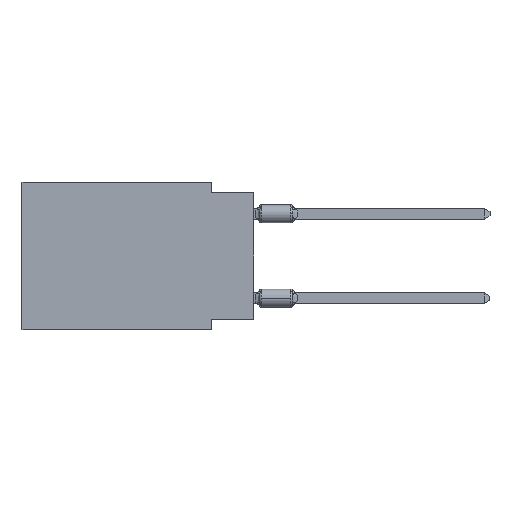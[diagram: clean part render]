
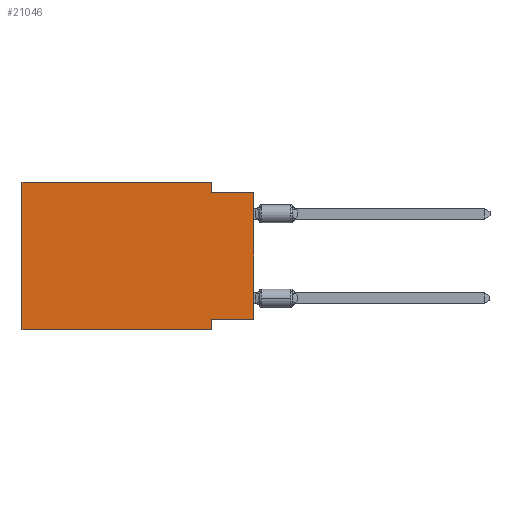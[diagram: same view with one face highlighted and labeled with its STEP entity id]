
A CAD part, left-side view. The second image highlights one B-rep face of the part: STEP entity #21046.
In plain terms, the highlighted planar face has unit normal (-1, 0, 0).
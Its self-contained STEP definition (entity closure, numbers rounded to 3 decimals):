
#267 = DIRECTION ( 'NONE',  ( 0., 1., 0. ) ) ;
#552 = EDGE_CURVE ( 'NONE', #5822, #3791, #19128, .T. ) ;
#1053 = LINE ( 'NONE', #17339, #16073 ) ;
#1590 = LINE ( 'NONE', #17991, #16207 ) ;
#1640 = VERTEX_POINT ( 'NONE', #14277 ) ;
#1796 = EDGE_CURVE ( 'NONE', #1640, #10874, #2358, .T. ) ;
#1816 = EDGE_CURVE ( 'NONE', #7917, #1640, #7277, .T. ) ;
#1916 = ORIENTED_EDGE ( 'NONE', *, *, #3583, .F. ) ;
#2358 = LINE ( 'NONE', #20168, #6768 ) ;
#2678 = VECTOR ( 'NONE', #6138, 1000. ) ;
#3006 = ORIENTED_EDGE ( 'NONE', *, *, #10089, .F. ) ;
#3583 = EDGE_CURVE ( 'NONE', #10874, #5408, #1053, .T. ) ;
#3791 = VERTEX_POINT ( 'NONE', #18504 ) ;
#3959 = FACE_OUTER_BOUND ( 'NONE', #9034, .T. ) ;
#4939 = LINE ( 'NONE', #11391, #18967 ) ;
#5405 = VECTOR ( 'NONE', #8885, 1000. ) ;
#5408 = VERTEX_POINT ( 'NONE', #6044 ) ;
#5555 = CARTESIAN_POINT ( 'NONE',  ( 0., 13.97, 0. ) ) ;
#5822 = VERTEX_POINT ( 'NONE', #7434 ) ;
#5949 = VECTOR ( 'NONE', #267, 1000. ) ;
#6044 = CARTESIAN_POINT ( 'NONE',  ( 0., 2.54, -0.635 ) ) ;
#6049 = CARTESIAN_POINT ( 'NONE',  ( 0., 2.54, -8.255 ) ) ;
#6138 = DIRECTION ( 'NONE',  ( 0., 0., 1. ) ) ;
#6193 = DIRECTION ( 'NONE',  ( 1., 0., 0. ) ) ;
#6768 = VECTOR ( 'NONE', #18866, 1000. ) ;
#6989 = VERTEX_POINT ( 'NONE', #12054 ) ;
#7099 = ORIENTED_EDGE ( 'NONE', *, *, #16585, .T. ) ;
#7277 = LINE ( 'NONE', #5555, #5405 ) ;
#7434 = CARTESIAN_POINT ( 'NONE',  ( 0., 0., -8.255 ) ) ;
#7748 = CARTESIAN_POINT ( 'NONE',  ( 0., 0., 0. ) ) ;
#7917 = VERTEX_POINT ( 'NONE', #17046 ) ;
#8117 = DIRECTION ( 'NONE',  ( 0., 0., -1. ) ) ;
#8775 = CARTESIAN_POINT ( 'NONE',  ( 0., 2.54, 0. ) ) ;
#8819 = LINE ( 'NONE', #11829, #5949 ) ;
#8885 = DIRECTION ( 'NONE',  ( 0., 0., 1. ) ) ;
#9034 = EDGE_LOOP ( 'NONE', ( #11129, #19531, #1916, #21090, #13071, #7099, #3006, #9657 ) ) ;
#9657 = ORIENTED_EDGE ( 'NONE', *, *, #12760, .F. ) ;
#10089 = EDGE_CURVE ( 'NONE', #17240, #6989, #1590, .T. ) ;
#10495 = PLANE ( 'NONE',  #18399 ) ;
#10874 = VERTEX_POINT ( 'NONE', #8775 ) ;
#11129 = ORIENTED_EDGE ( 'NONE', *, *, #552, .T. ) ;
#11179 = VECTOR ( 'NONE', #15325, 1000. ) ;
#11391 = CARTESIAN_POINT ( 'NONE',  ( 0., 13.97, -8.89 ) ) ;
#11829 = CARTESIAN_POINT ( 'NONE',  ( 0., 0., -8.255 ) ) ;
#12054 = CARTESIAN_POINT ( 'NONE',  ( 0., 2.54, -8.89 ) ) ;
#12520 = DIRECTION ( 'NONE',  ( 0., 0., -1. ) ) ;
#12760 = EDGE_CURVE ( 'NONE', #5822, #17240, #8819, .T. ) ;
#13071 = ORIENTED_EDGE ( 'NONE', *, *, #1816, .F. ) ;
#13396 = LINE ( 'NONE', #13610, #11179 ) ;
#13610 = CARTESIAN_POINT ( 'NONE',  ( 0., 0., -0.635 ) ) ;
#14277 = CARTESIAN_POINT ( 'NONE',  ( 0., 13.97, 0. ) ) ;
#14611 = DIRECTION ( 'NONE',  ( 0., -1., 0. ) ) ;
#14743 = EDGE_CURVE ( 'NONE', #5408, #3791, #13396, .T. ) ;
#15325 = DIRECTION ( 'NONE',  ( 0., -1., 0. ) ) ;
#16073 = VECTOR ( 'NONE', #12520, 1000. ) ;
#16207 = VECTOR ( 'NONE', #8117, 1000. ) ;
#16585 = EDGE_CURVE ( 'NONE', #7917, #6989, #4939, .T. ) ;
#17046 = CARTESIAN_POINT ( 'NONE',  ( 0., 13.97, -8.89 ) ) ;
#17240 = VERTEX_POINT ( 'NONE', #6049 ) ;
#17339 = CARTESIAN_POINT ( 'NONE',  ( 0., 2.54, 0. ) ) ;
#17991 = CARTESIAN_POINT ( 'NONE',  ( 0., 2.54, -8.89 ) ) ;
#18399 = AXIS2_PLACEMENT_3D ( 'NONE', #19082, #6193, #20906 ) ;
#18504 = CARTESIAN_POINT ( 'NONE',  ( 0., 0., -0.635 ) ) ;
#18866 = DIRECTION ( 'NONE',  ( 0., -1., 0. ) ) ;
#18967 = VECTOR ( 'NONE', #14611, 1000. ) ;
#19082 = CARTESIAN_POINT ( 'NONE',  ( 0., 13.97, 0. ) ) ;
#19128 = LINE ( 'NONE', #7748, #2678 ) ;
#19531 = ORIENTED_EDGE ( 'NONE', *, *, #14743, .F. ) ;
#20168 = CARTESIAN_POINT ( 'NONE',  ( 0., 13.97, 0. ) ) ;
#20906 = DIRECTION ( 'NONE',  ( 0., 0., -1. ) ) ;
#21046 = ADVANCED_FACE ( 'NONE', ( #3959 ), #10495, .F. ) ;
#21090 = ORIENTED_EDGE ( 'NONE', *, *, #1796, .F. ) ;
